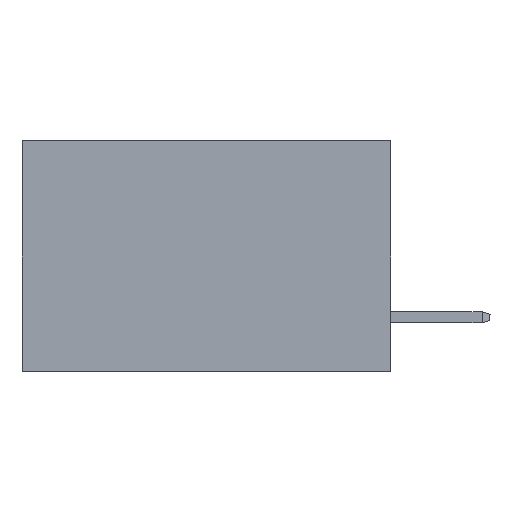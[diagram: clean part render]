
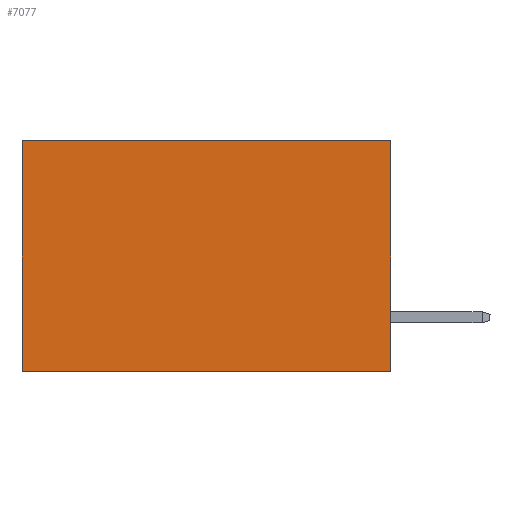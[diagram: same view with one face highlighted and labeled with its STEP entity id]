
A CAD part, left-side view. The second image highlights one B-rep face of the part: STEP entity #7077.
In plain terms, the highlighted planar face has unit normal (-1, 0, 0).
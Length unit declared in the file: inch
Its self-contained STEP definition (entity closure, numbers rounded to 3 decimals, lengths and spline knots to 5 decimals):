
#1 = AXIS2_PLACEMENT_3D ( 'NONE', #8874, #1961, #14700 ) ;
#375 = DIRECTION ( 'NONE',  ( 0., 0., -1. ) ) ;
#431 = LINE ( 'NONE', #12973, #14444 ) ;
#1214 = ORIENTED_EDGE ( 'NONE', *, *, #14788, .T. ) ;
#1961 = DIRECTION ( 'NONE',  ( 1., 0., 0. ) ) ;
#2011 = FACE_OUTER_BOUND ( 'NONE', #12136, .T. ) ;
#2323 = VECTOR ( 'NONE', #13887, 39.37008 ) ;
#2330 = ORIENTED_EDGE ( 'NONE', *, *, #8533, .F. ) ;
#2506 = CARTESIAN_POINT ( 'NONE',  ( 0.2875, 0., -0.375 ) ) ;
#3183 = VERTEX_POINT ( 'NONE', #7925 ) ;
#3295 = PLANE ( 'NONE',  #1 ) ;
#5169 = EDGE_CURVE ( 'NONE', #3183, #8306, #431, .T. ) ;
#5299 = LINE ( 'NONE', #10296, #12854 ) ;
#5757 = VERTEX_POINT ( 'NONE', #6474 ) ;
#5976 = CARTESIAN_POINT ( 'NONE',  ( 0.2875, 0.6, -0.375 ) ) ;
#6474 = CARTESIAN_POINT ( 'NONE',  ( 0.2875, 0.6, -0.375 ) ) ;
#6944 = DIRECTION ( 'NONE',  ( 0., 1., 0. ) ) ;
#7077 = ADVANCED_FACE ( 'NONE', ( #2011 ), #3295, .F. ) ;
#7925 = CARTESIAN_POINT ( 'NONE',  ( 0.2875, 0., 0. ) ) ;
#8040 = CARTESIAN_POINT ( 'NONE',  ( 0.2875, 0., -0.375 ) ) ;
#8306 = VERTEX_POINT ( 'NONE', #2506 ) ;
#8533 = EDGE_CURVE ( 'NONE', #8306, #5757, #10215, .T. ) ;
#8599 = VERTEX_POINT ( 'NONE', #12411 ) ;
#8874 = CARTESIAN_POINT ( 'NONE',  ( 0.2875, 0., -0.375 ) ) ;
#10215 = LINE ( 'NONE', #8040, #2323 ) ;
#10296 = CARTESIAN_POINT ( 'NONE',  ( 0.2875, 0., 0. ) ) ;
#10933 = ORIENTED_EDGE ( 'NONE', *, *, #5169, .F. ) ;
#10951 = LINE ( 'NONE', #5976, #13999 ) ;
#11355 = EDGE_CURVE ( 'NONE', #3183, #8599, #5299, .T. ) ;
#11864 = DIRECTION ( 'NONE',  ( 0., 0., -1. ) ) ;
#12136 = EDGE_LOOP ( 'NONE', ( #1214, #2330, #10933, #14809 ) ) ;
#12411 = CARTESIAN_POINT ( 'NONE',  ( 0.2875, 0.6, 0. ) ) ;
#12854 = VECTOR ( 'NONE', #6944, 39.37008 ) ;
#12973 = CARTESIAN_POINT ( 'NONE',  ( 0.2875, 0., -0.375 ) ) ;
#13887 = DIRECTION ( 'NONE',  ( 0., 1., 0. ) ) ;
#13999 = VECTOR ( 'NONE', #11864, 39.37008 ) ;
#14444 = VECTOR ( 'NONE', #375, 39.37008 ) ;
#14700 = DIRECTION ( 'NONE',  ( 0., 0., -1. ) ) ;
#14788 = EDGE_CURVE ( 'NONE', #8599, #5757, #10951, .T. ) ;
#14809 = ORIENTED_EDGE ( 'NONE', *, *, #11355, .T. ) ;
